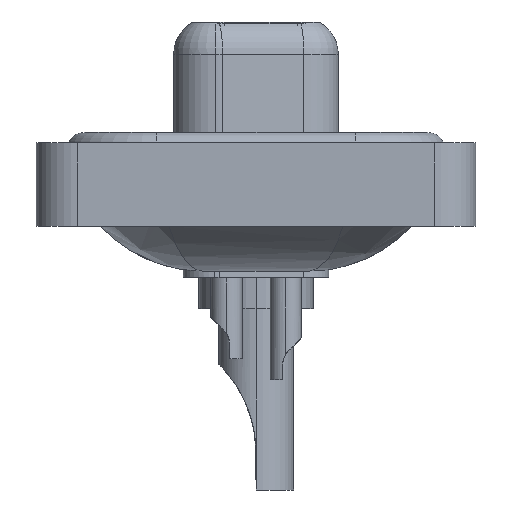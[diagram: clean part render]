
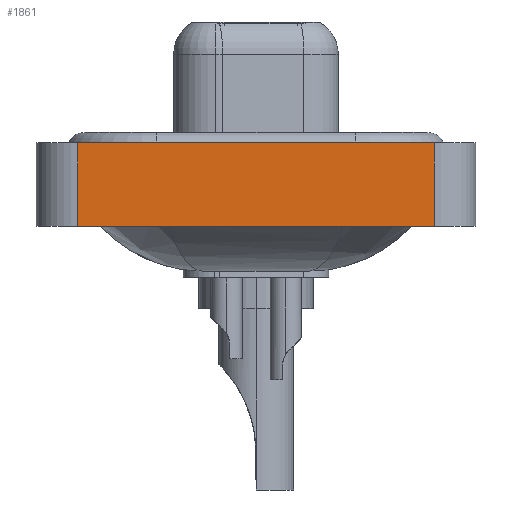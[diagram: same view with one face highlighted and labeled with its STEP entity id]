
A CAD part, left-side view. The second image highlights one B-rep face of the part: STEP entity #1861.
In plain terms, the highlighted planar face has unit normal (-1, 0, 0).
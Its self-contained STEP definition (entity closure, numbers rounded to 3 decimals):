
#43 = VERTEX_POINT ( 'NONE', #14414 ) ;
#227 = CARTESIAN_POINT ( 'NONE',  ( -7.25, -8.55, 0.4 ) ) ;
#272 = LINE ( 'NONE', #18257, #3364 ) ;
#1040 = DIRECTION ( 'NONE',  ( 0., 0., 1. ) ) ;
#1106 = DIRECTION ( 'NONE',  ( 0., 0., 1. ) ) ;
#1861 = ADVANCED_FACE ( 'NONE', ( #4939 ), #11209, .T. ) ;
#2823 = ORIENTED_EDGE ( 'NONE', *, *, #4212, .F. ) ;
#3364 = VECTOR ( 'NONE', #20244, 1000. ) ;
#3401 = DIRECTION ( 'NONE',  ( -1., 0., 0. ) ) ;
#4212 = EDGE_CURVE ( 'NONE', #43, #9959, #10443, .T. ) ;
#4687 = CARTESIAN_POINT ( 'NONE',  ( -7.25, 8.55, 0.4 ) ) ;
#4939 = FACE_OUTER_BOUND ( 'NONE', #19126, .T. ) ;
#4957 = DIRECTION ( 'NONE',  ( 0., -1., 0. ) ) ;
#6170 = EDGE_CURVE ( 'NONE', #43, #20187, #18989, .T. ) ;
#8246 = DIRECTION ( 'NONE',  ( 0., -1., 0. ) ) ;
#9088 = VECTOR ( 'NONE', #4957, 1000. ) ;
#9219 = CARTESIAN_POINT ( 'NONE',  ( -7.25, -8.55, -3.6 ) ) ;
#9926 = VERTEX_POINT ( 'NONE', #12295 ) ;
#9959 = VERTEX_POINT ( 'NONE', #4687 ) ;
#10220 = AXIS2_PLACEMENT_3D ( 'NONE', #17434, #3401, #1040 ) ;
#10443 = LINE ( 'NONE', #15322, #12951 ) ;
#10704 = ORIENTED_EDGE ( 'NONE', *, *, #15914, .T. ) ;
#11209 = PLANE ( 'NONE',  #10220 ) ;
#11231 = CARTESIAN_POINT ( 'NONE',  ( -7.25, -8.55, -3.6 ) ) ;
#12295 = CARTESIAN_POINT ( 'NONE',  ( -7.25, -8.55, 0.4 ) ) ;
#12653 = VECTOR ( 'NONE', #8246, 1000. ) ;
#12951 = VECTOR ( 'NONE', #1106, 1000. ) ;
#14262 = LINE ( 'NONE', #227, #12653 ) ;
#14414 = CARTESIAN_POINT ( 'NONE',  ( -7.25, 8.55, -3.6 ) ) ;
#15322 = CARTESIAN_POINT ( 'NONE',  ( -7.25, 8.55, -3.6 ) ) ;
#15914 = EDGE_CURVE ( 'NONE', #20187, #9926, #272, .T. ) ;
#16102 = ORIENTED_EDGE ( 'NONE', *, *, #18273, .F. ) ;
#17434 = CARTESIAN_POINT ( 'NONE',  ( -7.25, -8.55, -3.6 ) ) ;
#18063 = ORIENTED_EDGE ( 'NONE', *, *, #6170, .T. ) ;
#18257 = CARTESIAN_POINT ( 'NONE',  ( -7.25, -8.55, -3.6 ) ) ;
#18273 = EDGE_CURVE ( 'NONE', #9959, #9926, #14262, .T. ) ;
#18989 = LINE ( 'NONE', #11231, #9088 ) ;
#19126 = EDGE_LOOP ( 'NONE', ( #10704, #16102, #2823, #18063 ) ) ;
#20187 = VERTEX_POINT ( 'NONE', #9219 ) ;
#20244 = DIRECTION ( 'NONE',  ( 0., 0., 1. ) ) ;
